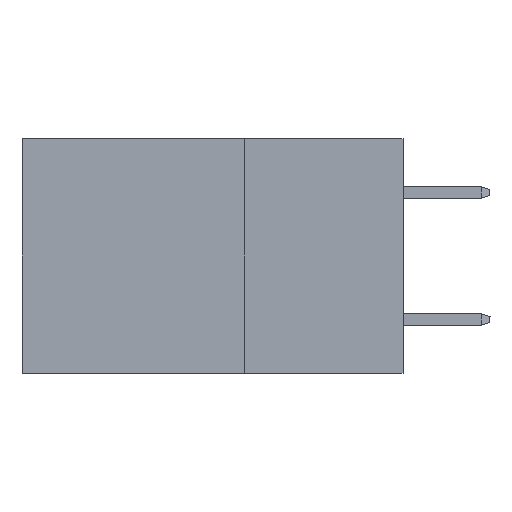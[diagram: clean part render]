
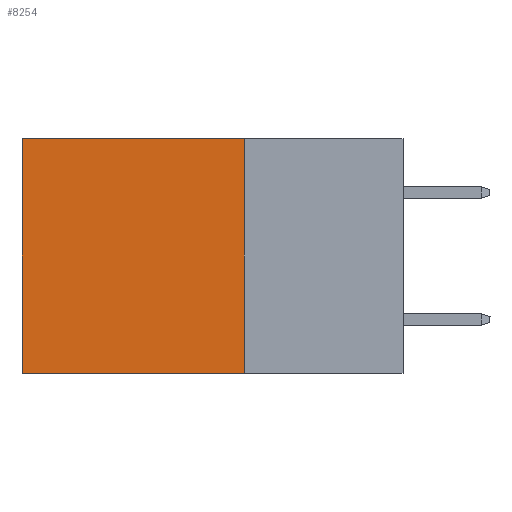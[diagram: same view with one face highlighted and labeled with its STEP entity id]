
A CAD part, left-side view. The second image highlights one B-rep face of the part: STEP entity #8254.
In plain terms, the highlighted planar face has unit normal (-1, 0, 0).
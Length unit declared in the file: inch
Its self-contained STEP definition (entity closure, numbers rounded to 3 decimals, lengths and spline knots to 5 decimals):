
#83 = DIRECTION ( 'NONE',  ( 0., 1., 0. ) ) ;
#139 = ORIENTED_EDGE ( 'NONE', *, *, #484, .F. ) ;
#368 = CARTESIAN_POINT ( 'NONE',  ( 0.2875, 0.25, 0. ) ) ;
#484 = EDGE_CURVE ( 'NONE', #26691, #17186, #16727, .T. ) ;
#930 = VERTEX_POINT ( 'NONE', #22512 ) ;
#1165 = VERTEX_POINT ( 'NONE', #6407 ) ;
#1453 = DIRECTION ( 'NONE',  ( 0., 0., -1. ) ) ;
#4750 = DIRECTION ( 'NONE',  ( 0., 1., 0. ) ) ;
#6393 = ORIENTED_EDGE ( 'NONE', *, *, #23747, .T. ) ;
#6407 = CARTESIAN_POINT ( 'NONE',  ( 0.2875, 0.6, -0.37 ) ) ;
#6609 = PLANE ( 'NONE',  #13877 ) ;
#7576 = CARTESIAN_POINT ( 'NONE',  ( 0.2875, 0.6, 0. ) ) ;
#7856 = ORIENTED_EDGE ( 'NONE', *, *, #28181, .T. ) ;
#8254 = ADVANCED_FACE ( 'NONE', ( #15628 ), #6609, .F. ) ;
#9036 = DIRECTION ( 'NONE',  ( 1., 0., 0. ) ) ;
#9627 = CARTESIAN_POINT ( 'NONE',  ( 0.2875, 0.25, 0. ) ) ;
#10880 = CARTESIAN_POINT ( 'NONE',  ( 0.2875, 0.25, 0. ) ) ;
#11033 = DIRECTION ( 'NONE',  ( 0., 0., -1. ) ) ;
#11738 = VECTOR ( 'NONE', #24012, 39.37008 ) ;
#13746 = VECTOR ( 'NONE', #83, 39.37008 ) ;
#13877 = AXIS2_PLACEMENT_3D ( 'NONE', #10880, #9036, #11033 ) ;
#14306 = LINE ( 'NONE', #21070, #13746 ) ;
#15628 = FACE_OUTER_BOUND ( 'NONE', #20818, .T. ) ;
#16008 = EDGE_CURVE ( 'NONE', #17186, #1165, #14306, .T. ) ;
#16727 = LINE ( 'NONE', #368, #11738 ) ;
#17186 = VERTEX_POINT ( 'NONE', #28508 ) ;
#20221 = CARTESIAN_POINT ( 'NONE',  ( 0.2875, 0.25, 0. ) ) ;
#20818 = EDGE_LOOP ( 'NONE', ( #6393, #28788, #139, #7856 ) ) ;
#21070 = CARTESIAN_POINT ( 'NONE',  ( 0.2875, 0.25, -0.37 ) ) ;
#21974 = VECTOR ( 'NONE', #4750, 39.37008 ) ;
#22512 = CARTESIAN_POINT ( 'NONE',  ( 0.2875, 0.6, 0. ) ) ;
#23644 = LINE ( 'NONE', #9627, #21974 ) ;
#23747 = EDGE_CURVE ( 'NONE', #930, #1165, #28636, .T. ) ;
#23872 = VECTOR ( 'NONE', #1453, 39.37008 ) ;
#24012 = DIRECTION ( 'NONE',  ( 0., 0., -1. ) ) ;
#26691 = VERTEX_POINT ( 'NONE', #20221 ) ;
#28181 = EDGE_CURVE ( 'NONE', #26691, #930, #23644, .T. ) ;
#28508 = CARTESIAN_POINT ( 'NONE',  ( 0.2875, 0.25, -0.37 ) ) ;
#28636 = LINE ( 'NONE', #7576, #23872 ) ;
#28788 = ORIENTED_EDGE ( 'NONE', *, *, #16008, .F. ) ;
